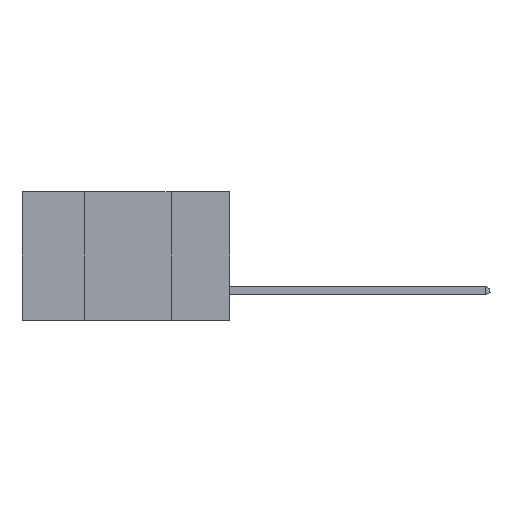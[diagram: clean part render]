
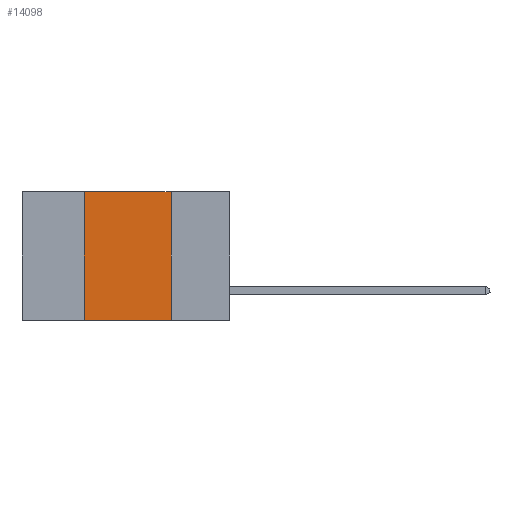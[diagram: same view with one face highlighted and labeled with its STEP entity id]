
A CAD part, left-side view. The second image highlights one B-rep face of the part: STEP entity #14098.
In plain terms, the highlighted planar face has unit normal (-1, 0, 0).
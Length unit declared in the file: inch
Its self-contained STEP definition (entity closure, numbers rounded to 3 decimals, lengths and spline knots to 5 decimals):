
#1351 = ORIENTED_EDGE ( 'NONE', *, *, #12743, .F. ) ;
#2626 = CARTESIAN_POINT ( 'NONE',  ( 0., 0.42, 0. ) ) ;
#3248 = ORIENTED_EDGE ( 'NONE', *, *, #18222, .F. ) ;
#3577 = EDGE_LOOP ( 'NONE', ( #1351, #19089, #3248, #14431 ) ) ;
#3603 = DIRECTION ( 'NONE',  ( 0., 0., -1. ) ) ;
#4082 = CARTESIAN_POINT ( 'NONE',  ( 0., 0.6, 0. ) ) ;
#4944 = VECTOR ( 'NONE', #19743, 39.37008 ) ;
#6397 = DIRECTION ( 'NONE',  ( 0., 0., -1. ) ) ;
#8615 = CARTESIAN_POINT ( 'NONE',  ( 0., 0.17, 0. ) ) ;
#8632 = EDGE_CURVE ( 'NONE', #9027, #10727, #17571, .T. ) ;
#9027 = VERTEX_POINT ( 'NONE', #12712 ) ;
#10500 = LINE ( 'NONE', #8615, #23106 ) ;
#10727 = VERTEX_POINT ( 'NONE', #28649 ) ;
#10843 = VECTOR ( 'NONE', #21958, 39.37008 ) ;
#11970 = FACE_OUTER_BOUND ( 'NONE', #3577, .T. ) ;
#12712 = CARTESIAN_POINT ( 'NONE',  ( 0., 0.42, -0.37 ) ) ;
#12743 = EDGE_CURVE ( 'NONE', #22185, #10727, #10500, .T. ) ;
#14098 = ADVANCED_FACE ( 'NONE', ( #11970 ), #23375, .F. ) ;
#14431 = ORIENTED_EDGE ( 'NONE', *, *, #8632, .T. ) ;
#16629 = EDGE_CURVE ( 'NONE', #28544, #22185, #24150, .T. ) ;
#16773 = DIRECTION ( 'NONE',  ( 1., 0., 0. ) ) ;
#17226 = DIRECTION ( 'NONE',  ( 0., 0., 1. ) ) ;
#17571 = LINE ( 'NONE', #24165, #10843 ) ;
#18222 = EDGE_CURVE ( 'NONE', #9027, #28544, #28803, .T. ) ;
#19089 = ORIENTED_EDGE ( 'NONE', *, *, #16629, .F. ) ;
#19709 = CARTESIAN_POINT ( 'NONE',  ( 0., 0.42, 0. ) ) ;
#19743 = DIRECTION ( 'NONE',  ( 0., -1., 0. ) ) ;
#20878 = CARTESIAN_POINT ( 'NONE',  ( 0., 0.6, 0. ) ) ;
#21958 = DIRECTION ( 'NONE',  ( 0., -1., 0. ) ) ;
#22185 = VERTEX_POINT ( 'NONE', #22576 ) ;
#22576 = CARTESIAN_POINT ( 'NONE',  ( 0., 0.17, 0. ) ) ;
#23106 = VECTOR ( 'NONE', #6397, 39.37008 ) ;
#23375 = PLANE ( 'NONE',  #23610 ) ;
#23610 = AXIS2_PLACEMENT_3D ( 'NONE', #20878, #16773, #3603 ) ;
#23709 = VECTOR ( 'NONE', #17226, 39.37008 ) ;
#24150 = LINE ( 'NONE', #4082, #4944 ) ;
#24165 = CARTESIAN_POINT ( 'NONE',  ( 0., 0.6, -0.37 ) ) ;
#28544 = VERTEX_POINT ( 'NONE', #2626 ) ;
#28649 = CARTESIAN_POINT ( 'NONE',  ( 0., 0.17, -0.37 ) ) ;
#28803 = LINE ( 'NONE', #19709, #23709 ) ;
